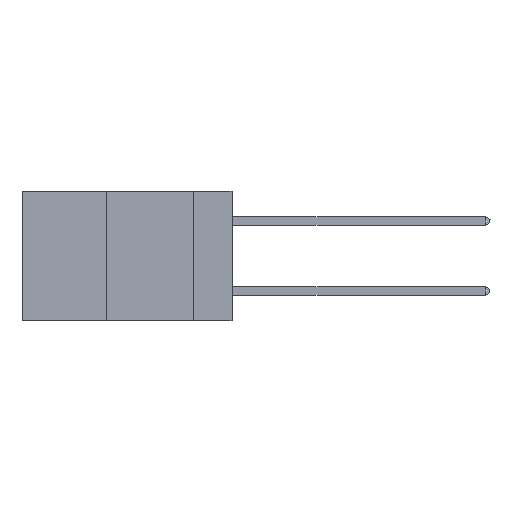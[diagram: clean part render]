
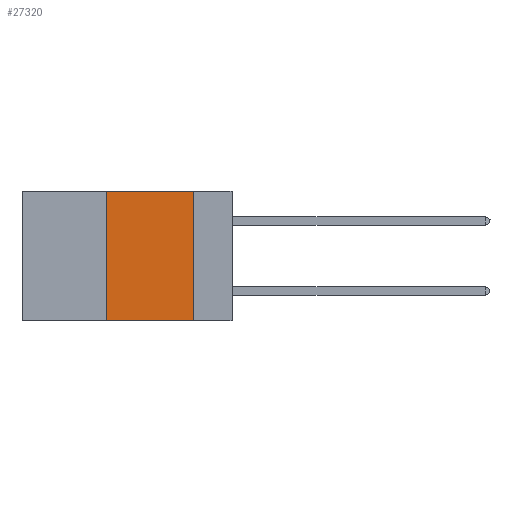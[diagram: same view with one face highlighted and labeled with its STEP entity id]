
A CAD part, left-side view. The second image highlights one B-rep face of the part: STEP entity #27320.
In plain terms, the highlighted planar face has unit normal (-1, 0, 0).
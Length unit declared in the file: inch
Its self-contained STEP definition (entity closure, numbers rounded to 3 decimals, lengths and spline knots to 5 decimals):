
#1004 = VERTEX_POINT ( 'NONE', #26008 ) ;
#1301 = CARTESIAN_POINT ( 'NONE',  ( 0., 0.36, 0. ) ) ;
#1687 = EDGE_CURVE ( 'NONE', #1004, #30237, #5736, .T. ) ;
#2085 = EDGE_CURVE ( 'NONE', #7894, #28783, #8236, .T. ) ;
#2313 = ORIENTED_EDGE ( 'NONE', *, *, #1687, .F. ) ;
#2565 = VECTOR ( 'NONE', #15819, 39.37008 ) ;
#3648 = VECTOR ( 'NONE', #11901, 39.37008 ) ;
#4320 = ORIENTED_EDGE ( 'NONE', *, *, #2085, .F. ) ;
#5736 = LINE ( 'NONE', #28083, #19402 ) ;
#7640 = CARTESIAN_POINT ( 'NONE',  ( 0., 0.6, 0. ) ) ;
#7894 = VERTEX_POINT ( 'NONE', #34227 ) ;
#8236 = LINE ( 'NONE', #8790, #3648 ) ;
#8790 = CARTESIAN_POINT ( 'NONE',  ( 0., 0.11, 0. ) ) ;
#9269 = ORIENTED_EDGE ( 'NONE', *, *, #9630, .T. ) ;
#9630 = EDGE_CURVE ( 'NONE', #1004, #28783, #29731, .T. ) ;
#9844 = DIRECTION ( 'NONE',  ( 0., -1., 0. ) ) ;
#9850 = FACE_OUTER_BOUND ( 'NONE', #21351, .T. ) ;
#11901 = DIRECTION ( 'NONE',  ( 0., 0., -1. ) ) ;
#13869 = DIRECTION ( 'NONE',  ( 0., 0., -1. ) ) ;
#15819 = DIRECTION ( 'NONE',  ( 0., -1., 0. ) ) ;
#16989 = VECTOR ( 'NONE', #9844, 39.37008 ) ;
#18153 = ORIENTED_EDGE ( 'NONE', *, *, #25949, .F. ) ;
#19402 = VECTOR ( 'NONE', #22600, 39.37008 ) ;
#20552 = AXIS2_PLACEMENT_3D ( 'NONE', #7640, #22104, #13869 ) ;
#21351 = EDGE_LOOP ( 'NONE', ( #4320, #18153, #2313, #9269 ) ) ;
#22104 = DIRECTION ( 'NONE',  ( 1., 0., 0. ) ) ;
#22600 = DIRECTION ( 'NONE',  ( 0., 0., 1. ) ) ;
#25949 = EDGE_CURVE ( 'NONE', #30237, #7894, #34557, .T. ) ;
#26008 = CARTESIAN_POINT ( 'NONE',  ( 0., 0.36, -0.37 ) ) ;
#27320 = ADVANCED_FACE ( 'NONE', ( #9850 ), #33083, .F. ) ;
#27519 = CARTESIAN_POINT ( 'NONE',  ( 0., 0.6, -0.37 ) ) ;
#27641 = CARTESIAN_POINT ( 'NONE',  ( 0., 0.11, -0.37 ) ) ;
#28083 = CARTESIAN_POINT ( 'NONE',  ( 0., 0.36, 0. ) ) ;
#28783 = VERTEX_POINT ( 'NONE', #27641 ) ;
#29731 = LINE ( 'NONE', #27519, #2565 ) ;
#30237 = VERTEX_POINT ( 'NONE', #1301 ) ;
#32358 = CARTESIAN_POINT ( 'NONE',  ( 0., 0.6, 0. ) ) ;
#33083 = PLANE ( 'NONE',  #20552 ) ;
#34227 = CARTESIAN_POINT ( 'NONE',  ( 0., 0.11, 0. ) ) ;
#34557 = LINE ( 'NONE', #32358, #16989 ) ;
